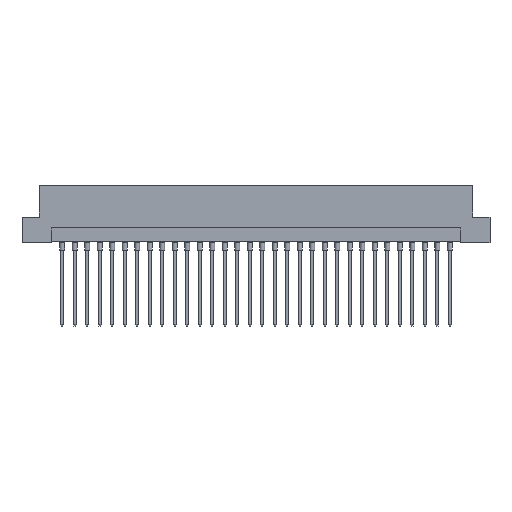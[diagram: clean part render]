
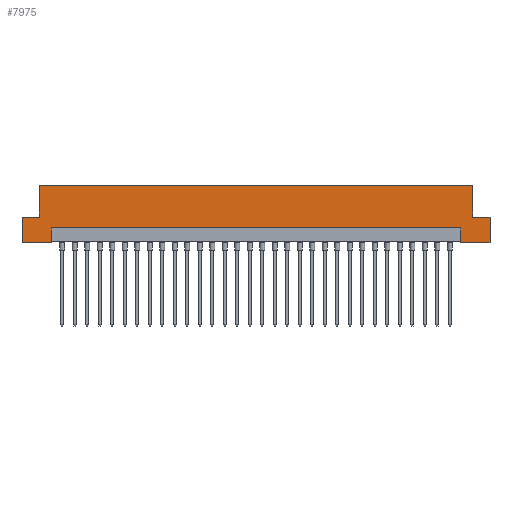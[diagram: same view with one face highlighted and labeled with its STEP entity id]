
A CAD part, front view. The second image highlights one B-rep face of the part: STEP entity #7975.
In plain terms, the highlighted planar face has unit normal (0, -1, 0).
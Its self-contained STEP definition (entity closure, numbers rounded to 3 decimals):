
#251 = DIRECTION ( 'NONE',  ( 0., 0., 1. ) ) ;
#339 = EDGE_CURVE ( 'NONE', #12769, #6248, #8430, .T. ) ;
#756 = LINE ( 'NONE', #12925, #5668 ) ;
#1140 = DIRECTION ( 'NONE',  ( 1., 0., 0. ) ) ;
#1333 = LINE ( 'NONE', #5280, #7591 ) ;
#1398 = DIRECTION ( 'NONE',  ( 1., 0., 0. ) ) ;
#1418 = EDGE_CURVE ( 'NONE', #7724, #9159, #11299, .T. ) ;
#2269 = CARTESIAN_POINT ( 'NONE',  ( 47.5, -4.3, 5.2 ) ) ;
#2353 = LINE ( 'NONE', #8325, #13019 ) ;
#2432 = DIRECTION ( 'NONE',  ( -1., 0., 0. ) ) ;
#2445 = LINE ( 'NONE', #9682, #2455 ) ;
#2455 = VECTOR ( 'NONE', #12729, 1000. ) ;
#2911 = EDGE_CURVE ( 'NONE', #9356, #9341, #1333, .T. ) ;
#2975 = VERTEX_POINT ( 'NONE', #2269 ) ;
#3764 = VERTEX_POINT ( 'NONE', #9033 ) ;
#3839 = DIRECTION ( 'NONE',  ( 1., 0., 0. ) ) ;
#4037 = ORIENTED_EDGE ( 'NONE', *, *, #10389, .T. ) ;
#4075 = EDGE_CURVE ( 'NONE', #2975, #9341, #2445, .T. ) ;
#4470 = LINE ( 'NONE', #6529, #6455 ) ;
#4754 = EDGE_CURVE ( 'NONE', #12604, #10276, #13033, .T. ) ;
#4962 = CARTESIAN_POINT ( 'NONE',  ( -47.5, -4.3, 5.2 ) ) ;
#5041 = CARTESIAN_POINT ( 'NONE',  ( -44., -4.3, 11.6 ) ) ;
#5246 = VERTEX_POINT ( 'NONE', #5568 ) ;
#5280 = CARTESIAN_POINT ( 'NONE',  ( 47.5, -4.3, 0. ) ) ;
#5324 = LINE ( 'NONE', #10622, #12816 ) ;
#5502 = FACE_OUTER_BOUND ( 'NONE', #11720, .T. ) ;
#5510 = ORIENTED_EDGE ( 'NONE', *, *, #4754, .T. ) ;
#5568 = CARTESIAN_POINT ( 'NONE',  ( 44., -4.3, 5.2 ) ) ;
#5578 = CARTESIAN_POINT ( 'NONE',  ( -41.6, -4.3, 0. ) ) ;
#5668 = VECTOR ( 'NONE', #3839, 1000. ) ;
#5949 = DIRECTION ( 'NONE',  ( 1., 0., 0. ) ) ;
#6097 = VECTOR ( 'NONE', #10531, 1000. ) ;
#6210 = DIRECTION ( 'NONE',  ( 0., 0., 1. ) ) ;
#6229 = PLANE ( 'NONE',  #7925 ) ;
#6248 = VERTEX_POINT ( 'NONE', #5578 ) ;
#6437 = EDGE_CURVE ( 'NONE', #9356, #10276, #10023, .T. ) ;
#6455 = VECTOR ( 'NONE', #9654, 1000. ) ;
#6457 = ORIENTED_EDGE ( 'NONE', *, *, #11478, .F. ) ;
#6458 = CARTESIAN_POINT ( 'NONE',  ( -44., -4.3, 5.2 ) ) ;
#6529 = CARTESIAN_POINT ( 'NONE',  ( -47.5, -4.3, 5.2 ) ) ;
#6539 = CARTESIAN_POINT ( 'NONE',  ( 44., -4.3, 5.2 ) ) ;
#6547 = VECTOR ( 'NONE', #9951, 1000. ) ;
#6582 = EDGE_CURVE ( 'NONE', #9645, #7724, #4470, .T. ) ;
#6915 = ORIENTED_EDGE ( 'NONE', *, *, #2911, .T. ) ;
#6958 = VECTOR ( 'NONE', #251, 1000. ) ;
#7295 = VECTOR ( 'NONE', #5949, 1000. ) ;
#7418 = CARTESIAN_POINT ( 'NONE',  ( 47.5, -4.3, 0. ) ) ;
#7420 = ORIENTED_EDGE ( 'NONE', *, *, #4075, .F. ) ;
#7591 = VECTOR ( 'NONE', #1398, 1000. ) ;
#7724 = VERTEX_POINT ( 'NONE', #10825 ) ;
#7925 = AXIS2_PLACEMENT_3D ( 'NONE', #11394, #9552, #2432 ) ;
#7940 = CARTESIAN_POINT ( 'NONE',  ( -41.6, -4.3, 0.2 ) ) ;
#7975 = ADVANCED_FACE ( 'NONE', ( #5502 ), #6229, .F. ) ;
#8325 = CARTESIAN_POINT ( 'NONE',  ( 47.5, -4.3, 5.2 ) ) ;
#8425 = EDGE_CURVE ( 'NONE', #5246, #2975, #2353, .T. ) ;
#8430 = LINE ( 'NONE', #9680, #8490 ) ;
#8490 = VECTOR ( 'NONE', #9444, 1000. ) ;
#8647 = ORIENTED_EDGE ( 'NONE', *, *, #10124, .F. ) ;
#8864 = EDGE_CURVE ( 'NONE', #9645, #12769, #5324, .T. ) ;
#8890 = LINE ( 'NONE', #7940, #6547 ) ;
#9033 = CARTESIAN_POINT ( 'NONE',  ( 44., -4.3, 11.6 ) ) ;
#9159 = VERTEX_POINT ( 'NONE', #5041 ) ;
#9341 = VERTEX_POINT ( 'NONE', #7418 ) ;
#9356 = VERTEX_POINT ( 'NONE', #9609 ) ;
#9444 = DIRECTION ( 'NONE',  ( 1., 0., 0. ) ) ;
#9552 = DIRECTION ( 'NONE',  ( 0., 1., 0. ) ) ;
#9609 = CARTESIAN_POINT ( 'NONE',  ( 41.6, -4.3, 0. ) ) ;
#9645 = VERTEX_POINT ( 'NONE', #4962 ) ;
#9654 = DIRECTION ( 'NONE',  ( 1., 0., 0. ) ) ;
#9680 = CARTESIAN_POINT ( 'NONE',  ( 47.5, -4.3, 0. ) ) ;
#9682 = CARTESIAN_POINT ( 'NONE',  ( 47.5, -4.3, 11.6 ) ) ;
#9805 = CARTESIAN_POINT ( 'NONE',  ( -41.6, -4.3, 3. ) ) ;
#9951 = DIRECTION ( 'NONE',  ( 0., 0., -1. ) ) ;
#10023 = LINE ( 'NONE', #11309, #13021 ) ;
#10049 = CARTESIAN_POINT ( 'NONE',  ( -41.6, -4.3, 3. ) ) ;
#10075 = CARTESIAN_POINT ( 'NONE',  ( 41.6, -4.3, 3. ) ) ;
#10124 = EDGE_CURVE ( 'NONE', #9159, #3764, #756, .T. ) ;
#10276 = VERTEX_POINT ( 'NONE', #10075 ) ;
#10389 = EDGE_CURVE ( 'NONE', #5246, #3764, #11576, .T. ) ;
#10531 = DIRECTION ( 'NONE',  ( 0., 0., 1. ) ) ;
#10536 = ORIENTED_EDGE ( 'NONE', *, *, #1418, .F. ) ;
#10562 = ORIENTED_EDGE ( 'NONE', *, *, #6582, .F. ) ;
#10592 = ORIENTED_EDGE ( 'NONE', *, *, #339, .T. ) ;
#10622 = CARTESIAN_POINT ( 'NONE',  ( -47.5, -4.3, 11.6 ) ) ;
#10825 = CARTESIAN_POINT ( 'NONE',  ( -44., -4.3, 5.2 ) ) ;
#11230 = CARTESIAN_POINT ( 'NONE',  ( -47.5, -4.3, 0. ) ) ;
#11240 = ORIENTED_EDGE ( 'NONE', *, *, #8425, .F. ) ;
#11299 = LINE ( 'NONE', #6458, #6958 ) ;
#11309 = CARTESIAN_POINT ( 'NONE',  ( 41.6, -4.3, 0.2 ) ) ;
#11394 = CARTESIAN_POINT ( 'NONE',  ( 47.5, -4.3, 11.6 ) ) ;
#11478 = EDGE_CURVE ( 'NONE', #12604, #6248, #8890, .T. ) ;
#11576 = LINE ( 'NONE', #6539, #6097 ) ;
#11720 = EDGE_LOOP ( 'NONE', ( #5510, #11995, #6915, #7420, #11240, #4037, #8647, #10536, #10562, #12214, #10592, #6457 ) ) ;
#11995 = ORIENTED_EDGE ( 'NONE', *, *, #6437, .F. ) ;
#12214 = ORIENTED_EDGE ( 'NONE', *, *, #8864, .T. ) ;
#12600 = DIRECTION ( 'NONE',  ( 0., 0., -1. ) ) ;
#12604 = VERTEX_POINT ( 'NONE', #10049 ) ;
#12729 = DIRECTION ( 'NONE',  ( 0., 0., -1. ) ) ;
#12769 = VERTEX_POINT ( 'NONE', #11230 ) ;
#12816 = VECTOR ( 'NONE', #12600, 1000. ) ;
#12925 = CARTESIAN_POINT ( 'NONE',  ( 47.5, -4.3, 11.6 ) ) ;
#13019 = VECTOR ( 'NONE', #1140, 1000. ) ;
#13021 = VECTOR ( 'NONE', #6210, 1000. ) ;
#13033 = LINE ( 'NONE', #9805, #7295 ) ;
